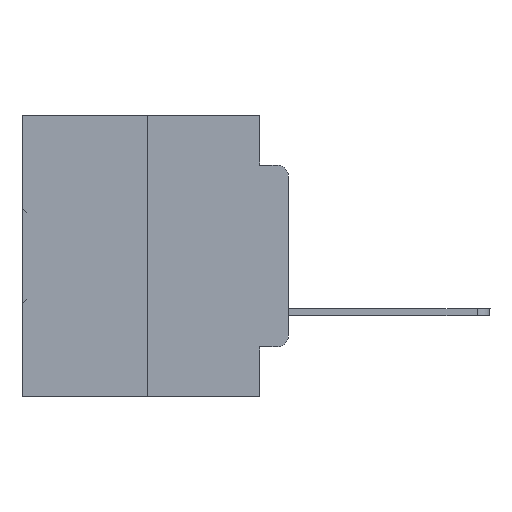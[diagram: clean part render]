
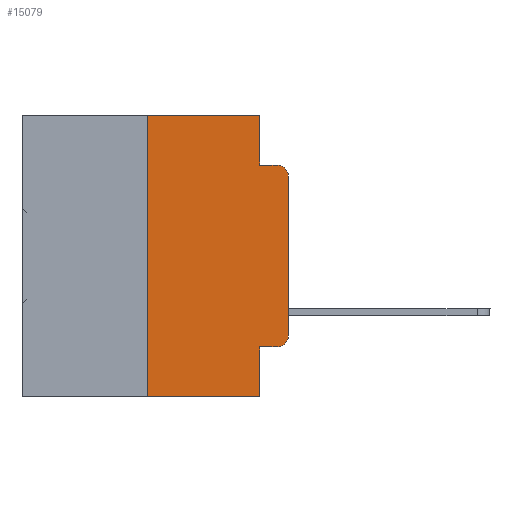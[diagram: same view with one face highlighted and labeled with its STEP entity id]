
A CAD part, left-side view. The second image highlights one B-rep face of the part: STEP entity #15079.
In plain terms, the highlighted planar face has unit normal (-1, 0, 0).
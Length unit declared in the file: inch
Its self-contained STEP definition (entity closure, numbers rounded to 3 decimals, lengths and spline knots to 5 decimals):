
#652 = VECTOR ( 'NONE', #9156, 39.37008 ) ;
#997 = VERTEX_POINT ( 'NONE', #27710 ) ;
#2158 = EDGE_CURVE ( 'NONE', #5829, #17867, #2196, .T. ) ;
#2196 = LINE ( 'NONE', #25956, #33002 ) ;
#2236 = ORIENTED_EDGE ( 'NONE', *, *, #21136, .F. ) ;
#2890 = EDGE_LOOP ( 'NONE', ( #21112, #7055, #22190, #13420, #2236, #24136, #3748, #24096, #21692, #8089 ) ) ;
#2900 = CARTESIAN_POINT ( 'NONE',  ( 0., 0.051, -0.4115 ) ) ;
#3475 = CARTESIAN_POINT ( 'NONE',  ( 0., 0.473, 0. ) ) ;
#3748 = ORIENTED_EDGE ( 'NONE', *, *, #27387, .T. ) ;
#4698 = VERTEX_POINT ( 'NONE', #4743 ) ;
#4743 = CARTESIAN_POINT ( 'NONE',  ( 0., 0., -0.1085 ) ) ;
#5829 = VERTEX_POINT ( 'NONE', #2900 ) ;
#5951 = EDGE_CURVE ( 'NONE', #17291, #12206, #30152, .T. ) ;
#6123 = DIRECTION ( 'NONE',  ( -1., 0., 0. ) ) ;
#6130 = EDGE_CURVE ( 'NONE', #4698, #12107, #13409, .T. ) ;
#6512 = CARTESIAN_POINT ( 'NONE',  ( 0., 0., -0.3915 ) ) ;
#7055 = ORIENTED_EDGE ( 'NONE', *, *, #6130, .T. ) ;
#7719 = LINE ( 'NONE', #11999, #12440 ) ;
#8089 = ORIENTED_EDGE ( 'NONE', *, *, #5951, .T. ) ;
#8322 = LINE ( 'NONE', #13234, #9660 ) ;
#8439 = AXIS2_PLACEMENT_3D ( 'NONE', #22385, #9148, #28471 ) ;
#8730 = PLANE ( 'NONE',  #14332 ) ;
#8893 = DIRECTION ( 'NONE',  ( 0., -1., 0. ) ) ;
#8991 = CARTESIAN_POINT ( 'NONE',  ( 0., 0.25, 0. ) ) ;
#9019 = CARTESIAN_POINT ( 'NONE',  ( 0., 0.051, 0. ) ) ;
#9148 = DIRECTION ( 'NONE',  ( -1., 0., 0. ) ) ;
#9156 = DIRECTION ( 'NONE',  ( 0., 0., 1. ) ) ;
#9411 = LINE ( 'NONE', #32951, #20206 ) ;
#9471 = LINE ( 'NONE', #32682, #19927 ) ;
#9660 = VECTOR ( 'NONE', #29604, 39.37008 ) ;
#10957 = LINE ( 'NONE', #16709, #24598 ) ;
#11167 = VERTEX_POINT ( 'NONE', #26189 ) ;
#11772 = LINE ( 'NONE', #27300, #652 ) ;
#11999 = CARTESIAN_POINT ( 'NONE',  ( 0., 0.051, -0.0885 ) ) ;
#12107 = VERTEX_POINT ( 'NONE', #12849 ) ;
#12206 = VERTEX_POINT ( 'NONE', #6512 ) ;
#12440 = VECTOR ( 'NONE', #23781, 39.37008 ) ;
#12849 = CARTESIAN_POINT ( 'NONE',  ( 0., 0.02, -0.0885 ) ) ;
#13214 = VECTOR ( 'NONE', #25245, 39.37008 ) ;
#13234 = CARTESIAN_POINT ( 'NONE',  ( 0., 0.051, -0.4115 ) ) ;
#13409 = CIRCLE ( 'NONE', #29553, 0.02 ) ;
#13420 = ORIENTED_EDGE ( 'NONE', *, *, #15649, .F. ) ;
#14332 = AXIS2_PLACEMENT_3D ( 'NONE', #3475, #16760, #27389 ) ;
#15079 = ADVANCED_FACE ( 'NONE', ( #21978 ), #8730, .F. ) ;
#15649 = EDGE_CURVE ( 'NONE', #11167, #27396, #24912, .T. ) ;
#16709 = CARTESIAN_POINT ( 'NONE',  ( 0., 0., 0. ) ) ;
#16760 = DIRECTION ( 'NONE',  ( 1., 0., 0. ) ) ;
#16777 = VERTEX_POINT ( 'NONE', #8991 ) ;
#17291 = VERTEX_POINT ( 'NONE', #20269 ) ;
#17867 = VERTEX_POINT ( 'NONE', #23368 ) ;
#18706 = CARTESIAN_POINT ( 'NONE',  ( 0., 0.02, -0.1085 ) ) ;
#19427 = CARTESIAN_POINT ( 'NONE',  ( 0., 0.051, -0.0885 ) ) ;
#19774 = EDGE_CURVE ( 'NONE', #12206, #4698, #10957, .T. ) ;
#19927 = VECTOR ( 'NONE', #27951, 39.37008 ) ;
#20206 = VECTOR ( 'NONE', #8893, 39.37008 ) ;
#20269 = CARTESIAN_POINT ( 'NONE',  ( 0., 0.02, -0.4115 ) ) ;
#21112 = ORIENTED_EDGE ( 'NONE', *, *, #19774, .T. ) ;
#21136 = EDGE_CURVE ( 'NONE', #16777, #11167, #9411, .T. ) ;
#21341 = EDGE_CURVE ( 'NONE', #5829, #17291, #8322, .T. ) ;
#21665 = EDGE_CURVE ( 'NONE', #27396, #12107, #7719, .T. ) ;
#21692 = ORIENTED_EDGE ( 'NONE', *, *, #21341, .T. ) ;
#21978 = FACE_OUTER_BOUND ( 'NONE', #2890, .T. ) ;
#22013 = DIRECTION ( 'NONE',  ( 0., 0., -1. ) ) ;
#22190 = ORIENTED_EDGE ( 'NONE', *, *, #21665, .F. ) ;
#22385 = CARTESIAN_POINT ( 'NONE',  ( 0., 0.02, -0.3915 ) ) ;
#23368 = CARTESIAN_POINT ( 'NONE',  ( 0., 0.051, -0.5 ) ) ;
#23781 = DIRECTION ( 'NONE',  ( 0., -1., 0. ) ) ;
#24096 = ORIENTED_EDGE ( 'NONE', *, *, #2158, .F. ) ;
#24136 = ORIENTED_EDGE ( 'NONE', *, *, #33094, .F. ) ;
#24598 = VECTOR ( 'NONE', #29427, 39.37008 ) ;
#24912 = LINE ( 'NONE', #9019, #13214 ) ;
#25245 = DIRECTION ( 'NONE',  ( 0., 0., -1. ) ) ;
#25774 = DIRECTION ( 'NONE',  ( 0., 0., -1. ) ) ;
#25956 = CARTESIAN_POINT ( 'NONE',  ( 0., 0.051, 0. ) ) ;
#26189 = CARTESIAN_POINT ( 'NONE',  ( 0., 0.051, 0. ) ) ;
#27300 = CARTESIAN_POINT ( 'NONE',  ( 0., 0.25, 0. ) ) ;
#27387 = EDGE_CURVE ( 'NONE', #997, #17867, #9471, .T. ) ;
#27389 = DIRECTION ( 'NONE',  ( 0., 0., -1. ) ) ;
#27396 = VERTEX_POINT ( 'NONE', #19427 ) ;
#27710 = CARTESIAN_POINT ( 'NONE',  ( 0., 0.25, -0.5 ) ) ;
#27951 = DIRECTION ( 'NONE',  ( 0., -1., 0. ) ) ;
#28471 = DIRECTION ( 'NONE',  ( 0., 0., -1. ) ) ;
#29427 = DIRECTION ( 'NONE',  ( 0., 0., 1. ) ) ;
#29553 = AXIS2_PLACEMENT_3D ( 'NONE', #18706, #6123, #22013 ) ;
#29604 = DIRECTION ( 'NONE',  ( 0., -1., 0. ) ) ;
#30152 = CIRCLE ( 'NONE', #8439, 0.02 ) ;
#32682 = CARTESIAN_POINT ( 'NONE',  ( 0., 0.473, -0.5 ) ) ;
#32951 = CARTESIAN_POINT ( 'NONE',  ( 0., 0.473, 0. ) ) ;
#33002 = VECTOR ( 'NONE', #25774, 39.37008 ) ;
#33094 = EDGE_CURVE ( 'NONE', #997, #16777, #11772, .T. ) ;
